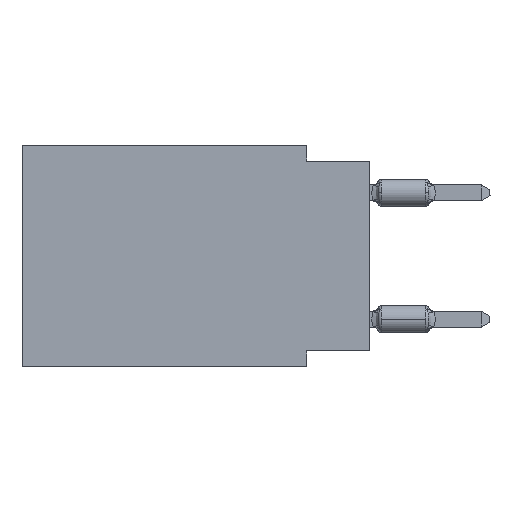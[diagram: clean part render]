
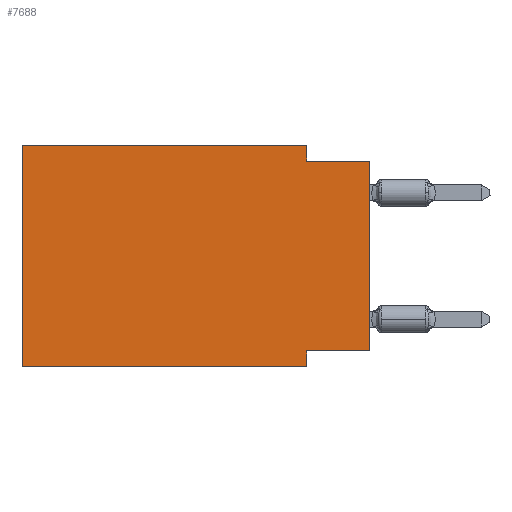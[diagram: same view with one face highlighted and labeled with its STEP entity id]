
A CAD part, left-side view. The second image highlights one B-rep face of the part: STEP entity #7688.
In plain terms, the highlighted planar face has unit normal (-1, 0, 0).
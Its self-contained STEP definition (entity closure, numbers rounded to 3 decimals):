
#13 = VECTOR ( 'NONE', #26572, 1000. ) ;
#148 = ORIENTED_EDGE ( 'NONE', *, *, #32045, .F. ) ;
#274 = VECTOR ( 'NONE', #19148, 1000. ) ;
#824 = VECTOR ( 'NONE', #19771, 1000. ) ;
#871 = ORIENTED_EDGE ( 'NONE', *, *, #16060, .F. ) ;
#925 = LINE ( 'NONE', #29480, #22466 ) ;
#3979 = VECTOR ( 'NONE', #16055, 1000. ) ;
#4101 = EDGE_CURVE ( 'NONE', #6035, #35361, #10890, .T. ) ;
#4332 = PLANE ( 'NONE',  #34581 ) ;
#4607 = DIRECTION ( 'NONE',  ( 0., -1., 0. ) ) ;
#5151 = CARTESIAN_POINT ( 'NONE',  ( 0., 13.97, -8.89 ) ) ;
#5286 = CARTESIAN_POINT ( 'NONE',  ( 0., 2.54, 0. ) ) ;
#5415 = CARTESIAN_POINT ( 'NONE',  ( 0., 13.97, 0. ) ) ;
#5497 = ORIENTED_EDGE ( 'NONE', *, *, #4101, .T. ) ;
#6035 = VERTEX_POINT ( 'NONE', #12690 ) ;
#6378 = DIRECTION ( 'NONE',  ( 0., -1., 0. ) ) ;
#7688 = ADVANCED_FACE ( 'NONE', ( #35469 ), #4332, .F. ) ;
#8601 = LINE ( 'NONE', #33830, #35337 ) ;
#8753 = VERTEX_POINT ( 'NONE', #5286 ) ;
#8915 = EDGE_CURVE ( 'NONE', #35796, #10762, #26961, .T. ) ;
#9188 = CARTESIAN_POINT ( 'NONE',  ( 0., 2.54, -8.89 ) ) ;
#9883 = CARTESIAN_POINT ( 'NONE',  ( 0., 13.97, 0. ) ) ;
#10482 = LINE ( 'NONE', #36243, #3979 ) ;
#10762 = VERTEX_POINT ( 'NONE', #23524 ) ;
#10880 = VERTEX_POINT ( 'NONE', #26873 ) ;
#10890 = LINE ( 'NONE', #5151, #23113 ) ;
#12157 = LINE ( 'NONE', #12723, #20920 ) ;
#12690 = CARTESIAN_POINT ( 'NONE',  ( 0., 13.97, -8.89 ) ) ;
#12723 = CARTESIAN_POINT ( 'NONE',  ( 0., 0., -8.255 ) ) ;
#14801 = ORIENTED_EDGE ( 'NONE', *, *, #17712, .F. ) ;
#15015 = DIRECTION ( 'NONE',  ( 0., 0., 1. ) ) ;
#15239 = CARTESIAN_POINT ( 'NONE',  ( 0., 13.97, 0. ) ) ;
#16055 = DIRECTION ( 'NONE',  ( 0., 0., -1. ) ) ;
#16060 = EDGE_CURVE ( 'NONE', #36176, #35361, #23283, .T. ) ;
#17547 = EDGE_CURVE ( 'NONE', #8753, #35796, #10482, .T. ) ;
#17712 = EDGE_CURVE ( 'NONE', #29291, #8753, #8601, .T. ) ;
#18433 = CARTESIAN_POINT ( 'NONE',  ( 0., 2.54, -8.255 ) ) ;
#18780 = DIRECTION ( 'NONE',  ( 0., 0., -1. ) ) ;
#18968 = CARTESIAN_POINT ( 'NONE',  ( 0., 0., -0.635 ) ) ;
#19148 = DIRECTION ( 'NONE',  ( 0., -1., 0. ) ) ;
#19771 = DIRECTION ( 'NONE',  ( 0., 0., -1. ) ) ;
#20920 = VECTOR ( 'NONE', #23463, 1000. ) ;
#21960 = EDGE_CURVE ( 'NONE', #10880, #10762, #925, .T. ) ;
#22466 = VECTOR ( 'NONE', #15015, 1000. ) ;
#23113 = VECTOR ( 'NONE', #4607, 1000. ) ;
#23277 = EDGE_CURVE ( 'NONE', #6035, #29291, #26013, .T. ) ;
#23283 = LINE ( 'NONE', #9188, #824 ) ;
#23463 = DIRECTION ( 'NONE',  ( 0., 1., 0. ) ) ;
#23524 = CARTESIAN_POINT ( 'NONE',  ( 0., 0., -0.635 ) ) ;
#24084 = CARTESIAN_POINT ( 'NONE',  ( 0., 2.54, -8.89 ) ) ;
#24150 = ORIENTED_EDGE ( 'NONE', *, *, #17547, .F. ) ;
#24387 = EDGE_LOOP ( 'NONE', ( #26564, #34533, #24150, #14801, #32581, #5497, #871, #148 ) ) ;
#26013 = LINE ( 'NONE', #15239, #13 ) ;
#26564 = ORIENTED_EDGE ( 'NONE', *, *, #21960, .T. ) ;
#26572 = DIRECTION ( 'NONE',  ( 0., 0., 1. ) ) ;
#26873 = CARTESIAN_POINT ( 'NONE',  ( 0., 0., -8.255 ) ) ;
#26961 = LINE ( 'NONE', #18968, #274 ) ;
#29291 = VERTEX_POINT ( 'NONE', #5415 ) ;
#29480 = CARTESIAN_POINT ( 'NONE',  ( 0., 0., 0. ) ) ;
#29773 = CARTESIAN_POINT ( 'NONE',  ( 0., 2.54, -0.635 ) ) ;
#32045 = EDGE_CURVE ( 'NONE', #10880, #36176, #12157, .T. ) ;
#32581 = ORIENTED_EDGE ( 'NONE', *, *, #23277, .F. ) ;
#33830 = CARTESIAN_POINT ( 'NONE',  ( 0., 13.97, 0. ) ) ;
#34533 = ORIENTED_EDGE ( 'NONE', *, *, #8915, .F. ) ;
#34581 = AXIS2_PLACEMENT_3D ( 'NONE', #9883, #35646, #18780 ) ;
#35337 = VECTOR ( 'NONE', #6378, 1000. ) ;
#35361 = VERTEX_POINT ( 'NONE', #24084 ) ;
#35469 = FACE_OUTER_BOUND ( 'NONE', #24387, .T. ) ;
#35646 = DIRECTION ( 'NONE',  ( 1., 0., 0. ) ) ;
#35796 = VERTEX_POINT ( 'NONE', #29773 ) ;
#36176 = VERTEX_POINT ( 'NONE', #18433 ) ;
#36243 = CARTESIAN_POINT ( 'NONE',  ( 0., 2.54, 0. ) ) ;
